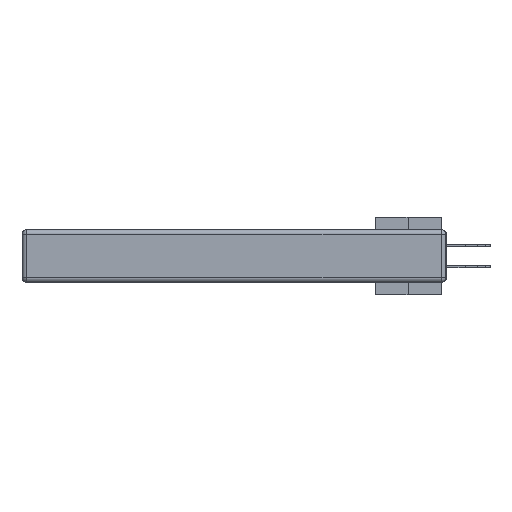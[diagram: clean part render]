
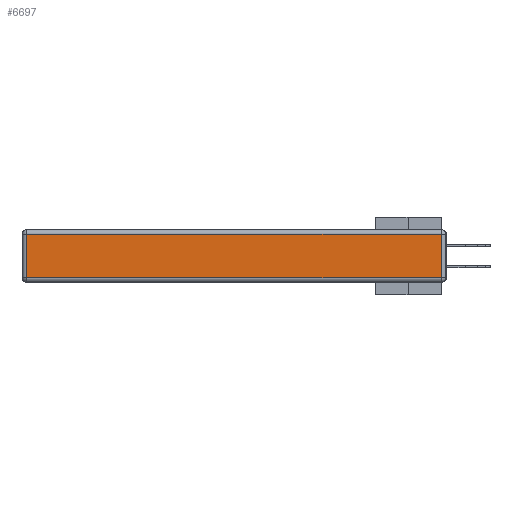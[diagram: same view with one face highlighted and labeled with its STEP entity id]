
A CAD part, left-side view. The second image highlights one B-rep face of the part: STEP entity #6697.
In plain terms, the highlighted planar face has unit normal (-1, 0, 0).
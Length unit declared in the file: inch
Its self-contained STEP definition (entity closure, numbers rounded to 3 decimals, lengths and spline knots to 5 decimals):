
#88 = LINE ( 'NONE', #547, #17372 ) ;
#547 = CARTESIAN_POINT ( 'NONE',  ( 0., 2.75, -0.03 ) ) ;
#4170 = LINE ( 'NONE', #7931, #8909 ) ;
#5430 = EDGE_LOOP ( 'NONE', ( #15592, #12664, #31304, #31096 ) ) ;
#5764 = CARTESIAN_POINT ( 'NONE',  ( 0., 2.72, -0.313 ) ) ;
#6697 = ADVANCED_FACE ( 'NONE', ( #21914 ), #23097, .T. ) ;
#7931 = CARTESIAN_POINT ( 'NONE',  ( 0., 2.72, -0.343 ) ) ;
#8909 = VECTOR ( 'NONE', #32787, 39.37008 ) ;
#9205 = EDGE_CURVE ( 'NONE', #13130, #31507, #88, .T. ) ;
#9436 = CARTESIAN_POINT ( 'NONE',  ( 0., 0., -0.313 ) ) ;
#9688 = AXIS2_PLACEMENT_3D ( 'NONE', #17442, #17806, #28814 ) ;
#10066 = VERTEX_POINT ( 'NONE', #15611 ) ;
#12664 = ORIENTED_EDGE ( 'NONE', *, *, #20132, .T. ) ;
#13130 = VERTEX_POINT ( 'NONE', #22835 ) ;
#13436 = LINE ( 'NONE', #9436, #32467 ) ;
#15413 = DIRECTION ( 'NONE',  ( 0., 0., 1. ) ) ;
#15592 = ORIENTED_EDGE ( 'NONE', *, *, #34792, .T. ) ;
#15611 = CARTESIAN_POINT ( 'NONE',  ( 0., 0.03, -0.313 ) ) ;
#17282 = DIRECTION ( 'NONE',  ( 0., -1., 0. ) ) ;
#17372 = VECTOR ( 'NONE', #22506, 39.37008 ) ;
#17442 = CARTESIAN_POINT ( 'NONE',  ( 0., 0., -0.343 ) ) ;
#17806 = DIRECTION ( 'NONE',  ( -1., 0., 0. ) ) ;
#18174 = LINE ( 'NONE', #29466, #22480 ) ;
#20132 = EDGE_CURVE ( 'NONE', #10066, #13130, #18174, .T. ) ;
#21914 = FACE_OUTER_BOUND ( 'NONE', #5430, .T. ) ;
#22480 = VECTOR ( 'NONE', #15413, 39.37008 ) ;
#22506 = DIRECTION ( 'NONE',  ( 0., 1., 0. ) ) ;
#22835 = CARTESIAN_POINT ( 'NONE',  ( 0., 0.03, -0.03 ) ) ;
#23097 = PLANE ( 'NONE',  #9688 ) ;
#24622 = VERTEX_POINT ( 'NONE', #5764 ) ;
#26327 = CARTESIAN_POINT ( 'NONE',  ( 0., 2.72, -0.03 ) ) ;
#26837 = EDGE_CURVE ( 'NONE', #31507, #24622, #4170, .T. ) ;
#28814 = DIRECTION ( 'NONE',  ( 0., 0., 1. ) ) ;
#29466 = CARTESIAN_POINT ( 'NONE',  ( 0., 0.03, -0.343 ) ) ;
#31096 = ORIENTED_EDGE ( 'NONE', *, *, #26837, .T. ) ;
#31304 = ORIENTED_EDGE ( 'NONE', *, *, #9205, .T. ) ;
#31507 = VERTEX_POINT ( 'NONE', #26327 ) ;
#32467 = VECTOR ( 'NONE', #17282, 39.37008 ) ;
#32787 = DIRECTION ( 'NONE',  ( 0., 0., -1. ) ) ;
#34792 = EDGE_CURVE ( 'NONE', #24622, #10066, #13436, .T. ) ;
